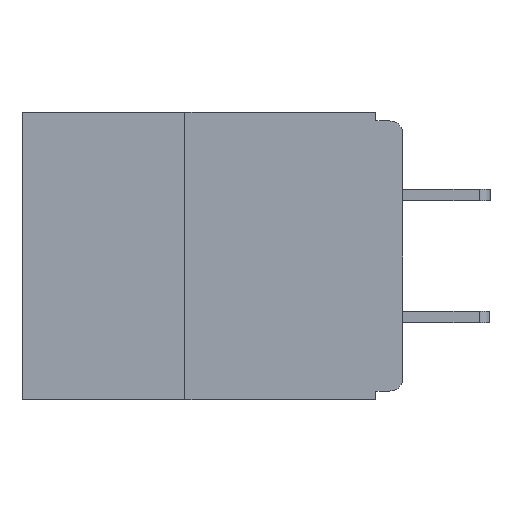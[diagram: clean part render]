
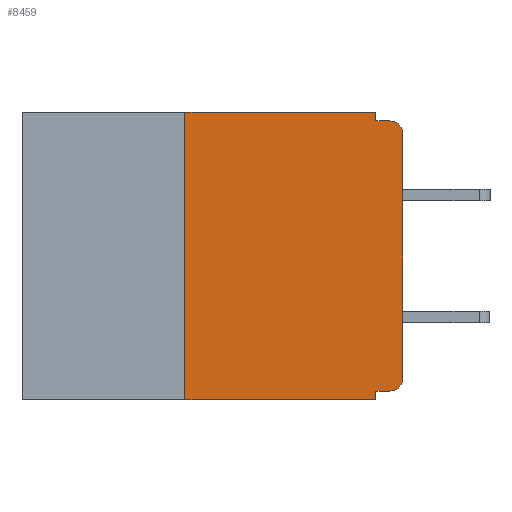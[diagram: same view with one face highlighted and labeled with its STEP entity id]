
A CAD part, left-side view. The second image highlights one B-rep face of the part: STEP entity #8459.
In plain terms, the highlighted planar face has unit normal (-1, 0, 0).
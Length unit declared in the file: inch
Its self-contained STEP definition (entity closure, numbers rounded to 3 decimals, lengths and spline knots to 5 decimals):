
#118 = CARTESIAN_POINT ( 'NONE',  ( 0., 0.437, 0. ) ) ;
#148 = EDGE_CURVE ( 'NONE', #3352, #12391, #8355, .T. ) ;
#270 = EDGE_CURVE ( 'NONE', #627, #7210, #4709, .T. ) ;
#369 = DIRECTION ( 'NONE',  ( 0., 0., 1. ) ) ;
#383 = ORIENTED_EDGE ( 'NONE', *, *, #270, .T. ) ;
#421 = ORIENTED_EDGE ( 'NONE', *, *, #148, .F. ) ;
#520 = CARTESIAN_POINT ( 'NONE',  ( 0., 0.25, -0.33 ) ) ;
#627 = VERTEX_POINT ( 'NONE', #4801 ) ;
#705 = LINE ( 'NONE', #2301, #11260 ) ;
#1029 = FACE_OUTER_BOUND ( 'NONE', #10112, .T. ) ;
#1396 = LINE ( 'NONE', #520, #9254 ) ;
#2224 = DIRECTION ( 'NONE',  ( 0., 0., -1. ) ) ;
#2301 = CARTESIAN_POINT ( 'NONE',  ( 0., 0.031, -0.33 ) ) ;
#2326 = ORIENTED_EDGE ( 'NONE', *, *, #8033, .F. ) ;
#2785 = ORIENTED_EDGE ( 'NONE', *, *, #5388, .F. ) ;
#3115 = CARTESIAN_POINT ( 'NONE',  ( 0., 0.015, -0.305 ) ) ;
#3284 = LINE ( 'NONE', #118, #8354 ) ;
#3320 = DIRECTION ( 'NONE',  ( -1., 0., 0. ) ) ;
#3352 = VERTEX_POINT ( 'NONE', #9585 ) ;
#3412 = CIRCLE ( 'NONE', #4866, 0.015 ) ;
#3582 = CARTESIAN_POINT ( 'NONE',  ( 0., 0., -0.305 ) ) ;
#3614 = DIRECTION ( 'NONE',  ( 0., 0., 1. ) ) ;
#3678 = CARTESIAN_POINT ( 'NONE',  ( 0., 0.015, -0.025 ) ) ;
#3732 = CARTESIAN_POINT ( 'NONE',  ( 0., 0.437, 0. ) ) ;
#3813 = CARTESIAN_POINT ( 'NONE',  ( 0., 0.015, -0.32 ) ) ;
#3815 = DIRECTION ( 'NONE',  ( 0., 1., 0. ) ) ;
#3860 = CARTESIAN_POINT ( 'NONE',  ( 0., 0., -0.32 ) ) ;
#3923 = VECTOR ( 'NONE', #12538, 39.37008 ) ;
#3935 = CARTESIAN_POINT ( 'NONE',  ( 0., 0.031, 0. ) ) ;
#4151 = DIRECTION ( 'NONE',  ( 0., 0., -1. ) ) ;
#4312 = EDGE_CURVE ( 'NONE', #5216, #3352, #3284, .T. ) ;
#4375 = CARTESIAN_POINT ( 'NONE',  ( 0., 0.031, -0.32 ) ) ;
#4537 = AXIS2_PLACEMENT_3D ( 'NONE', #3732, #7630, #7601 ) ;
#4554 = LINE ( 'NONE', #12683, #3923 ) ;
#4709 = LINE ( 'NONE', #6869, #5342 ) ;
#4801 = CARTESIAN_POINT ( 'NONE',  ( 0., 0.25, -0.33 ) ) ;
#4866 = AXIS2_PLACEMENT_3D ( 'NONE', #3678, #3320, #2224 ) ;
#5020 = ORIENTED_EDGE ( 'NONE', *, *, #4312, .F. ) ;
#5074 = AXIS2_PLACEMENT_3D ( 'NONE', #3115, #10195, #4151 ) ;
#5149 = CARTESIAN_POINT ( 'NONE',  ( 0., 0.015, -0.01 ) ) ;
#5216 = VERTEX_POINT ( 'NONE', #6786 ) ;
#5247 = CARTESIAN_POINT ( 'NONE',  ( 0., 0., -0.025 ) ) ;
#5342 = VECTOR ( 'NONE', #9004, 39.37008 ) ;
#5388 = EDGE_CURVE ( 'NONE', #12391, #6458, #4554, .T. ) ;
#5833 = ORIENTED_EDGE ( 'NONE', *, *, #8789, .F. ) ;
#6129 = EDGE_CURVE ( 'NONE', #10192, #6458, #3412, .T. ) ;
#6458 = VERTEX_POINT ( 'NONE', #5149 ) ;
#6459 = CIRCLE ( 'NONE', #5074, 0.015 ) ;
#6515 = VERTEX_POINT ( 'NONE', #3813 ) ;
#6541 = VERTEX_POINT ( 'NONE', #3582 ) ;
#6786 = CARTESIAN_POINT ( 'NONE',  ( 0., 0.25, 0. ) ) ;
#6869 = CARTESIAN_POINT ( 'NONE',  ( 0., 0.437, -0.33 ) ) ;
#7210 = VERTEX_POINT ( 'NONE', #8279 ) ;
#7535 = ORIENTED_EDGE ( 'NONE', *, *, #12209, .T. ) ;
#7601 = DIRECTION ( 'NONE',  ( 0., 0., -1. ) ) ;
#7630 = DIRECTION ( 'NONE',  ( 1., 0., 0. ) ) ;
#7691 = PLANE ( 'NONE',  #4537 ) ;
#8033 = EDGE_CURVE ( 'NONE', #627, #5216, #1396, .T. ) ;
#8122 = DIRECTION ( 'NONE',  ( 0., -1., 0. ) ) ;
#8279 = CARTESIAN_POINT ( 'NONE',  ( 0., 0.031, -0.33 ) ) ;
#8354 = VECTOR ( 'NONE', #8122, 39.37008 ) ;
#8355 = LINE ( 'NONE', #3935, #8670 ) ;
#8459 = ADVANCED_FACE ( 'NONE', ( #1029 ), #7691, .F. ) ;
#8670 = VECTOR ( 'NONE', #11476, 39.37008 ) ;
#8789 = EDGE_CURVE ( 'NONE', #11266, #7210, #705, .T. ) ;
#8910 = ORIENTED_EDGE ( 'NONE', *, *, #11395, .T. ) ;
#9004 = DIRECTION ( 'NONE',  ( 0., -1., 0. ) ) ;
#9207 = LINE ( 'NONE', #9691, #10143 ) ;
#9254 = VECTOR ( 'NONE', #369, 39.37008 ) ;
#9398 = LINE ( 'NONE', #3860, #11665 ) ;
#9467 = ORIENTED_EDGE ( 'NONE', *, *, #10356, .F. ) ;
#9514 = CARTESIAN_POINT ( 'NONE',  ( 0., 0.031, -0.01 ) ) ;
#9585 = CARTESIAN_POINT ( 'NONE',  ( 0., 0.031, 0. ) ) ;
#9691 = CARTESIAN_POINT ( 'NONE',  ( 0., 0., 0. ) ) ;
#10112 = EDGE_LOOP ( 'NONE', ( #8910, #13021, #2785, #421, #5020, #2326, #383, #5833, #9467, #7535 ) ) ;
#10143 = VECTOR ( 'NONE', #3614, 39.37008 ) ;
#10192 = VERTEX_POINT ( 'NONE', #5247 ) ;
#10195 = DIRECTION ( 'NONE',  ( -1., 0., 0. ) ) ;
#10356 = EDGE_CURVE ( 'NONE', #6515, #11266, #9398, .T. ) ;
#10428 = DIRECTION ( 'NONE',  ( 0., 0., -1. ) ) ;
#11260 = VECTOR ( 'NONE', #10428, 39.37008 ) ;
#11266 = VERTEX_POINT ( 'NONE', #4375 ) ;
#11395 = EDGE_CURVE ( 'NONE', #6541, #10192, #9207, .T. ) ;
#11476 = DIRECTION ( 'NONE',  ( 0., 0., -1. ) ) ;
#11665 = VECTOR ( 'NONE', #3815, 39.37008 ) ;
#12209 = EDGE_CURVE ( 'NONE', #6515, #6541, #6459, .T. ) ;
#12391 = VERTEX_POINT ( 'NONE', #9514 ) ;
#12538 = DIRECTION ( 'NONE',  ( 0., -1., 0. ) ) ;
#12683 = CARTESIAN_POINT ( 'NONE',  ( 0., 0., -0.01 ) ) ;
#13021 = ORIENTED_EDGE ( 'NONE', *, *, #6129, .T. ) ;
